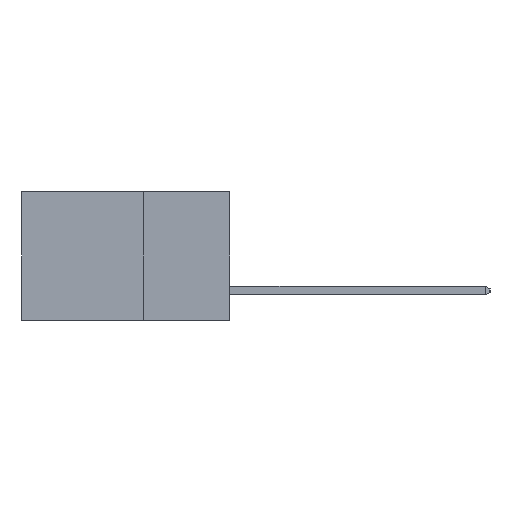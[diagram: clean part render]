
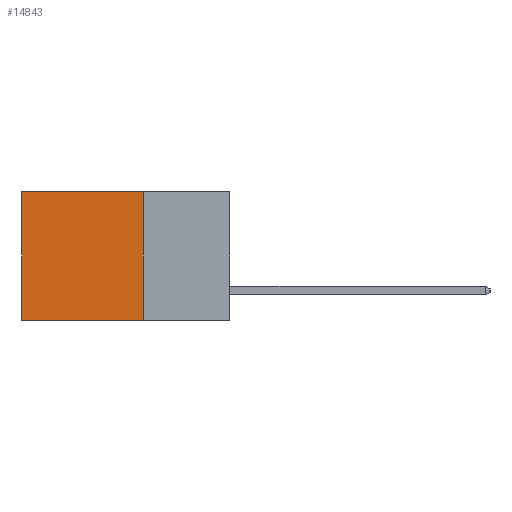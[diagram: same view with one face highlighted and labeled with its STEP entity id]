
A CAD part, left-side view. The second image highlights one B-rep face of the part: STEP entity #14843.
In plain terms, the highlighted planar face has unit normal (-1, 0, 0).
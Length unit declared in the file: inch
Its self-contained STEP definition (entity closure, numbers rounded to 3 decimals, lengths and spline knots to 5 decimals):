
#90 = CARTESIAN_POINT ( 'NONE',  ( 0.298, 0.6, -0.37 ) ) ;
#1079 = VECTOR ( 'NONE', #14533, 39.37008 ) ;
#1217 = ORIENTED_EDGE ( 'NONE', *, *, #14722, .F. ) ;
#1371 = ORIENTED_EDGE ( 'NONE', *, *, #14894, .T. ) ;
#1932 = EDGE_CURVE ( 'NONE', #5864, #11746, #7016, .T. ) ;
#2061 = VERTEX_POINT ( 'NONE', #5994 ) ;
#4279 = CARTESIAN_POINT ( 'NONE',  ( 0.298, 0.25, -0.37 ) ) ;
#4506 = PLANE ( 'NONE',  #13760 ) ;
#5258 = LINE ( 'NONE', #14687, #11048 ) ;
#5352 = VECTOR ( 'NONE', #12626, 39.37008 ) ;
#5540 = EDGE_CURVE ( 'NONE', #5864, #2061, #5258, .T. ) ;
#5864 = VERTEX_POINT ( 'NONE', #10706 ) ;
#5994 = CARTESIAN_POINT ( 'NONE',  ( 0.298, 0.25, -0.37 ) ) ;
#6127 = ORIENTED_EDGE ( 'NONE', *, *, #5540, .F. ) ;
#6909 = DIRECTION ( 'NONE',  ( 0., 0., -1. ) ) ;
#7016 = LINE ( 'NONE', #13687, #8093 ) ;
#8093 = VECTOR ( 'NONE', #8712, 39.37008 ) ;
#8454 = ORIENTED_EDGE ( 'NONE', *, *, #1932, .T. ) ;
#8712 = DIRECTION ( 'NONE',  ( 0., 1., 0. ) ) ;
#10204 = LINE ( 'NONE', #4279, #1079 ) ;
#10706 = CARTESIAN_POINT ( 'NONE',  ( 0.298, 0.25, 0. ) ) ;
#10938 = DIRECTION ( 'NONE',  ( 0., 0., -1. ) ) ;
#11048 = VECTOR ( 'NONE', #10938, 39.37008 ) ;
#11364 = VERTEX_POINT ( 'NONE', #90 ) ;
#11746 = VERTEX_POINT ( 'NONE', #14730 ) ;
#11815 = LINE ( 'NONE', #13714, #5352 ) ;
#12581 = CARTESIAN_POINT ( 'NONE',  ( 0.298, 0.25, 0. ) ) ;
#12626 = DIRECTION ( 'NONE',  ( 0., 0., -1. ) ) ;
#13667 = DIRECTION ( 'NONE',  ( 1., 0., 0. ) ) ;
#13687 = CARTESIAN_POINT ( 'NONE',  ( 0.298, 0.25, 0. ) ) ;
#13714 = CARTESIAN_POINT ( 'NONE',  ( 0.298, 0.6, 0. ) ) ;
#13760 = AXIS2_PLACEMENT_3D ( 'NONE', #12581, #13667, #6909 ) ;
#13911 = EDGE_LOOP ( 'NONE', ( #1371, #1217, #6127, #8454 ) ) ;
#14533 = DIRECTION ( 'NONE',  ( 0., 1., 0. ) ) ;
#14687 = CARTESIAN_POINT ( 'NONE',  ( 0.298, 0.25, 0. ) ) ;
#14722 = EDGE_CURVE ( 'NONE', #2061, #11364, #10204, .T. ) ;
#14730 = CARTESIAN_POINT ( 'NONE',  ( 0.298, 0.6, 0. ) ) ;
#14843 = ADVANCED_FACE ( 'NONE', ( #15054 ), #4506, .F. ) ;
#14894 = EDGE_CURVE ( 'NONE', #11746, #11364, #11815, .T. ) ;
#15054 = FACE_OUTER_BOUND ( 'NONE', #13911, .T. ) ;
